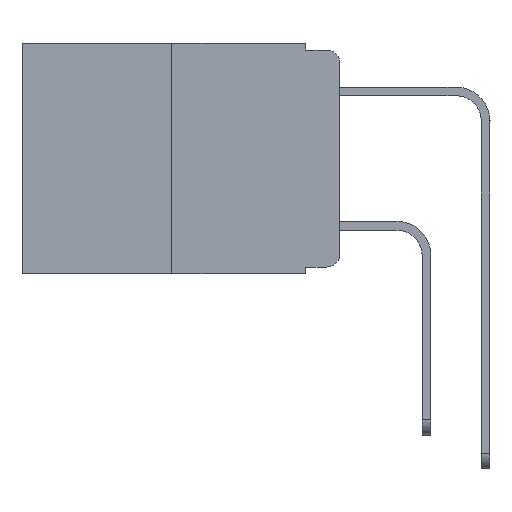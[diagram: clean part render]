
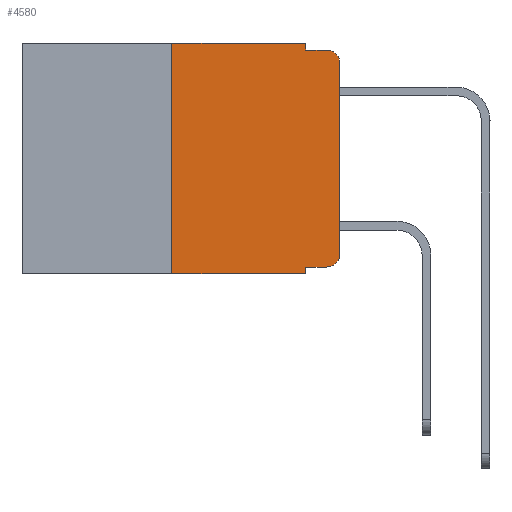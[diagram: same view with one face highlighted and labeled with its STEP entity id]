
A CAD part, left-side view. The second image highlights one B-rep face of the part: STEP entity #4580.
In plain terms, the highlighted planar face has unit normal (-1, 0, 0).
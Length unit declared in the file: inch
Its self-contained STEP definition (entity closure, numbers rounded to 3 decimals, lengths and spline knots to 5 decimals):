
#824 = VECTOR ( 'NONE', #11438, 39.37008 ) ;
#1998 = CARTESIAN_POINT ( 'NONE',  ( 0., 0.02, -0.333 ) ) ;
#2007 = CARTESIAN_POINT ( 'NONE',  ( 0., 0.051, -0.01 ) ) ;
#2219 = LINE ( 'NONE', #4027, #3539 ) ;
#2320 = EDGE_CURVE ( 'NONE', #13473, #24073, #17336, .T. ) ;
#2480 = EDGE_CURVE ( 'NONE', #21663, #24073, #4340, .T. ) ;
#2530 = ORIENTED_EDGE ( 'NONE', *, *, #18725, .F. ) ;
#2605 = DIRECTION ( 'NONE',  ( 0., 0., 1. ) ) ;
#2798 = ORIENTED_EDGE ( 'NONE', *, *, #17480, .T. ) ;
#2885 = VERTEX_POINT ( 'NONE', #3969 ) ;
#2967 = CARTESIAN_POINT ( 'NONE',  ( 0., 0.051, -0.343 ) ) ;
#2996 = CARTESIAN_POINT ( 'NONE',  ( 0., 0.02, -0.01 ) ) ;
#3488 = CARTESIAN_POINT ( 'NONE',  ( 0., 0.25, 0. ) ) ;
#3539 = VECTOR ( 'NONE', #11103, 39.37008 ) ;
#3731 = EDGE_CURVE ( 'NONE', #13473, #5527, #2219, .T. ) ;
#3969 = CARTESIAN_POINT ( 'NONE',  ( 0., 0.25, 0. ) ) ;
#4027 = CARTESIAN_POINT ( 'NONE',  ( 0., 0.051, -0.333 ) ) ;
#4340 = LINE ( 'NONE', #18882, #9074 ) ;
#4580 = ADVANCED_FACE ( 'NONE', ( #10726 ), #15077, .F. ) ;
#4852 = AXIS2_PLACEMENT_3D ( 'NONE', #22586, #5212, #18962 ) ;
#5094 = EDGE_CURVE ( 'NONE', #5527, #23050, #19186, .T. ) ;
#5212 = DIRECTION ( 'NONE',  ( 1., 0., 0. ) ) ;
#5509 = CARTESIAN_POINT ( 'NONE',  ( 0., 0., -0.313 ) ) ;
#5527 = VERTEX_POINT ( 'NONE', #1998 ) ;
#6145 = CARTESIAN_POINT ( 'NONE',  ( 0., 0.051, -0.333 ) ) ;
#6494 = CARTESIAN_POINT ( 'NONE',  ( 0., 0.02, -0.03 ) ) ;
#6689 = ORIENTED_EDGE ( 'NONE', *, *, #20021, .F. ) ;
#6896 = VECTOR ( 'NONE', #10465, 39.37008 ) ;
#7667 = CIRCLE ( 'NONE', #19599, 0.02 ) ;
#8291 = VECTOR ( 'NONE', #2605, 39.37008 ) ;
#8551 = DIRECTION ( 'NONE',  ( 0., 0., -1. ) ) ;
#9074 = VECTOR ( 'NONE', #22511, 39.37008 ) ;
#9671 = VERTEX_POINT ( 'NONE', #12833 ) ;
#9681 = CARTESIAN_POINT ( 'NONE',  ( 0., 0.051, 0. ) ) ;
#10180 = DIRECTION ( 'NONE',  ( 0., -1., 0. ) ) ;
#10465 = DIRECTION ( 'NONE',  ( 0., 0., -1. ) ) ;
#10726 = FACE_OUTER_BOUND ( 'NONE', #19348, .T. ) ;
#10793 = CARTESIAN_POINT ( 'NONE',  ( 0., 0.02, -0.313 ) ) ;
#10880 = DIRECTION ( 'NONE',  ( 0., -1., 0. ) ) ;
#11103 = DIRECTION ( 'NONE',  ( 0., -1., 0. ) ) ;
#11438 = DIRECTION ( 'NONE',  ( 0., 0., -1. ) ) ;
#11830 = VERTEX_POINT ( 'NONE', #9681 ) ;
#11947 = VERTEX_POINT ( 'NONE', #2996 ) ;
#12761 = DIRECTION ( 'NONE',  ( 0., 0., -1. ) ) ;
#12833 = CARTESIAN_POINT ( 'NONE',  ( 0., 0.051, -0.01 ) ) ;
#13473 = VERTEX_POINT ( 'NONE', #6145 ) ;
#13559 = EDGE_CURVE ( 'NONE', #16632, #11947, #7667, .T. ) ;
#13797 = ORIENTED_EDGE ( 'NONE', *, *, #2480, .T. ) ;
#14037 = ORIENTED_EDGE ( 'NONE', *, *, #13559, .T. ) ;
#14561 = CARTESIAN_POINT ( 'NONE',  ( 0., 0., 0. ) ) ;
#14639 = LINE ( 'NONE', #3488, #19757 ) ;
#14801 = CARTESIAN_POINT ( 'NONE',  ( 0., 0.473, 0. ) ) ;
#15077 = PLANE ( 'NONE',  #4852 ) ;
#15944 = ORIENTED_EDGE ( 'NONE', *, *, #5094, .T. ) ;
#16060 = VECTOR ( 'NONE', #10180, 39.37008 ) ;
#16632 = VERTEX_POINT ( 'NONE', #21540 ) ;
#16868 = ORIENTED_EDGE ( 'NONE', *, *, #2320, .F. ) ;
#17336 = LINE ( 'NONE', #22999, #6896 ) ;
#17480 = EDGE_CURVE ( 'NONE', #23050, #16632, #23679, .T. ) ;
#18642 = ORIENTED_EDGE ( 'NONE', *, *, #21276, .F. ) ;
#18725 = EDGE_CURVE ( 'NONE', #2885, #11830, #25366, .T. ) ;
#18882 = CARTESIAN_POINT ( 'NONE',  ( 0., 0.473, -0.343 ) ) ;
#18962 = DIRECTION ( 'NONE',  ( 0., 0., -1. ) ) ;
#19186 = CIRCLE ( 'NONE', #22644, 0.02 ) ;
#19348 = EDGE_LOOP ( 'NONE', ( #2798, #14037, #18642, #6689, #2530, #23370, #13797, #16868, #23095, #15944 ) ) ;
#19599 = AXIS2_PLACEMENT_3D ( 'NONE', #6494, #20165, #8551 ) ;
#19757 = VECTOR ( 'NONE', #24881, 39.37008 ) ;
#20021 = EDGE_CURVE ( 'NONE', #11830, #9671, #20615, .T. ) ;
#20165 = DIRECTION ( 'NONE',  ( -1., 0., 0. ) ) ;
#20615 = LINE ( 'NONE', #22917, #824 ) ;
#21131 = LINE ( 'NONE', #2007, #16060 ) ;
#21276 = EDGE_CURVE ( 'NONE', #9671, #11947, #21131, .T. ) ;
#21540 = CARTESIAN_POINT ( 'NONE',  ( 0., 0., -0.03 ) ) ;
#21663 = VERTEX_POINT ( 'NONE', #23834 ) ;
#22511 = DIRECTION ( 'NONE',  ( 0., -1., 0. ) ) ;
#22547 = EDGE_CURVE ( 'NONE', #21663, #2885, #14639, .T. ) ;
#22586 = CARTESIAN_POINT ( 'NONE',  ( 0., 0.473, 0. ) ) ;
#22644 = AXIS2_PLACEMENT_3D ( 'NONE', #10793, #24231, #12761 ) ;
#22917 = CARTESIAN_POINT ( 'NONE',  ( 0., 0.051, 0. ) ) ;
#22999 = CARTESIAN_POINT ( 'NONE',  ( 0., 0.051, 0. ) ) ;
#23050 = VERTEX_POINT ( 'NONE', #5509 ) ;
#23095 = ORIENTED_EDGE ( 'NONE', *, *, #3731, .T. ) ;
#23370 = ORIENTED_EDGE ( 'NONE', *, *, #22547, .F. ) ;
#23679 = LINE ( 'NONE', #14561, #8291 ) ;
#23834 = CARTESIAN_POINT ( 'NONE',  ( 0., 0.25, -0.343 ) ) ;
#24073 = VERTEX_POINT ( 'NONE', #2967 ) ;
#24207 = VECTOR ( 'NONE', #10880, 39.37008 ) ;
#24231 = DIRECTION ( 'NONE',  ( -1., 0., 0. ) ) ;
#24881 = DIRECTION ( 'NONE',  ( 0., 0., 1. ) ) ;
#25366 = LINE ( 'NONE', #14801, #24207 ) ;
